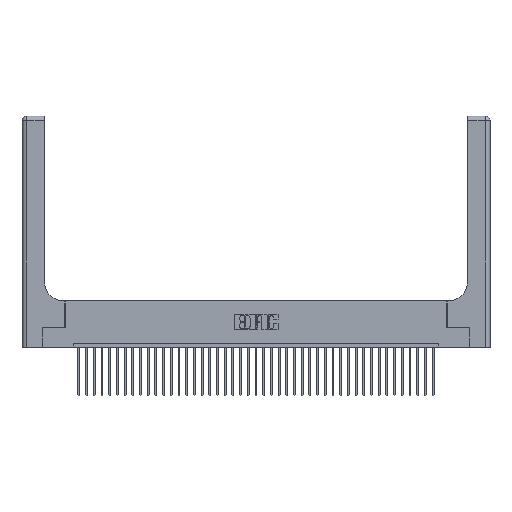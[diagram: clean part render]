
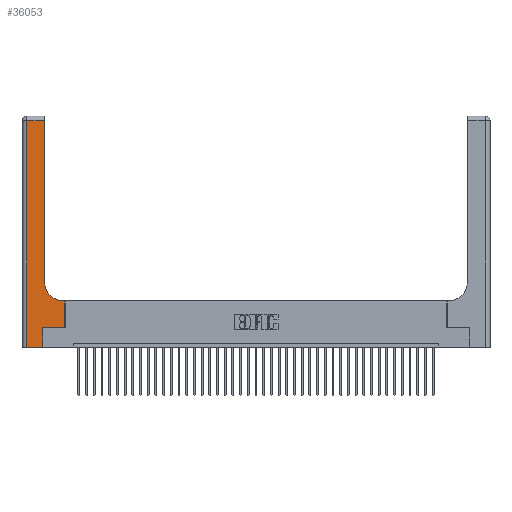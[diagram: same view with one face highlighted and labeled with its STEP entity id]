
A CAD part, top view. The second image highlights one B-rep face of the part: STEP entity #36053.
In plain terms, the highlighted planar face has unit normal (0, 0, 1).
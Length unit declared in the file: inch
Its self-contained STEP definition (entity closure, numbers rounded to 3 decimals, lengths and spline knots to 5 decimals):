
#49 = CARTESIAN_POINT ( 'NONE',  ( 0., 2.94, 0.37 ) ) ;
#161 = VERTEX_POINT ( 'NONE', #31166 ) ;
#651 = EDGE_CURVE ( 'NONE', #8113, #23962, #15244, .T. ) ;
#875 = CARTESIAN_POINT ( 'NONE',  ( 0., 0., 0.37 ) ) ;
#1107 = LINE ( 'NONE', #34322, #7401 ) ;
#2987 = DIRECTION ( 'NONE',  ( 1., 0., 0. ) ) ;
#3810 = LINE ( 'NONE', #9054, #38551 ) ;
#3890 = EDGE_CURVE ( 'NONE', #18270, #8113, #21351, .T. ) ;
#4877 = EDGE_CURVE ( 'NONE', #21331, #4894, #12464, .T. ) ;
#4894 = VERTEX_POINT ( 'NONE', #25846 ) ;
#6618 = CARTESIAN_POINT ( 'NONE',  ( 0.5415, 0.85, 0.37 ) ) ;
#6692 = DIRECTION ( 'NONE',  ( 1., 0., 0. ) ) ;
#6704 = CARTESIAN_POINT ( 'NONE',  ( 0.5585, 0.25, 0.37 ) ) ;
#7362 = VECTOR ( 'NONE', #6692, 39.37008 ) ;
#7401 = VECTOR ( 'NONE', #28544, 39.37008 ) ;
#8113 = VERTEX_POINT ( 'NONE', #14712 ) ;
#8853 = FACE_OUTER_BOUND ( 'NONE', #10346, .T. ) ;
#9054 = CARTESIAN_POINT ( 'NONE',  ( 0.269, 0.25, 0.37 ) ) ;
#9971 = VERTEX_POINT ( 'NONE', #36101 ) ;
#10346 = EDGE_LOOP ( 'NONE', ( #34549, #17338, #36298, #28625, #17336, #20316, #34508, #25698, #30585 ) ) ;
#10503 = DIRECTION ( 'NONE',  ( -1., 0., 0. ) ) ;
#11169 = CARTESIAN_POINT ( 'NONE',  ( 0.269, 0., 0.37 ) ) ;
#11776 = EDGE_CURVE ( 'NONE', #9971, #32318, #22780, .T. ) ;
#12464 = LINE ( 'NONE', #6704, #35665 ) ;
#12509 = CARTESIAN_POINT ( 'NONE',  ( 0.5585, 0.25, 0.37 ) ) ;
#13069 = DIRECTION ( 'NONE',  ( 0., 0., -1. ) ) ;
#14148 = DIRECTION ( 'NONE',  ( 0., 1., 0. ) ) ;
#14547 = CARTESIAN_POINT ( 'NONE',  ( 0.2915, 2.94, 0.37 ) ) ;
#14557 = VECTOR ( 'NONE', #10503, 39.37008 ) ;
#14712 = CARTESIAN_POINT ( 'NONE',  ( 0.06, 2.94, 0.37 ) ) ;
#15244 = LINE ( 'NONE', #39171, #17190 ) ;
#15920 = DIRECTION ( 'NONE',  ( 0., 1., 0. ) ) ;
#17190 = VECTOR ( 'NONE', #17551, 39.37008 ) ;
#17336 = ORIENTED_EDGE ( 'NONE', *, *, #11776, .T. ) ;
#17338 = ORIENTED_EDGE ( 'NONE', *, *, #3890, .T. ) ;
#17534 = CARTESIAN_POINT ( 'NONE',  ( 0.269, 0.25, 0.37 ) ) ;
#17551 = DIRECTION ( 'NONE',  ( 0., -1., 0. ) ) ;
#18270 = VERTEX_POINT ( 'NONE', #14547 ) ;
#19774 = CARTESIAN_POINT ( 'NONE',  ( 0., 3., 0.37 ) ) ;
#20312 = VECTOR ( 'NONE', #22445, 39.37008 ) ;
#20316 = ORIENTED_EDGE ( 'NONE', *, *, #36431, .T. ) ;
#20877 = EDGE_CURVE ( 'NONE', #23962, #9971, #24330, .T. ) ;
#21331 = VERTEX_POINT ( 'NONE', #12509 ) ;
#21351 = LINE ( 'NONE', #49, #14557 ) ;
#22445 = DIRECTION ( 'NONE',  ( 0., 1., 0. ) ) ;
#22780 = LINE ( 'NONE', #11169, #35804 ) ;
#22971 = AXIS2_PLACEMENT_3D ( 'NONE', #6618, #13069, #28205 ) ;
#23962 = VERTEX_POINT ( 'NONE', #29622 ) ;
#24330 = LINE ( 'NONE', #875, #7362 ) ;
#24387 = EDGE_CURVE ( 'NONE', #4894, #36514, #1107, .T. ) ;
#25698 = ORIENTED_EDGE ( 'NONE', *, *, #24387, .T. ) ;
#25846 = CARTESIAN_POINT ( 'NONE',  ( 0.5585, 0.6, 0.37 ) ) ;
#26446 = EDGE_CURVE ( 'NONE', #161, #18270, #38524, .T. ) ;
#27929 = CARTESIAN_POINT ( 'NONE',  ( 0.5415, 0.6, 0.37 ) ) ;
#28205 = DIRECTION ( 'NONE',  ( 1., 0., 0. ) ) ;
#28544 = DIRECTION ( 'NONE',  ( -1., 0., 0. ) ) ;
#28625 = ORIENTED_EDGE ( 'NONE', *, *, #20877, .T. ) ;
#28633 = PLANE ( 'NONE',  #38048 ) ;
#28774 = DIRECTION ( 'NONE',  ( 0., 0., -1. ) ) ;
#28905 = CARTESIAN_POINT ( 'NONE',  ( 0.2915, 3., 0.37 ) ) ;
#29622 = CARTESIAN_POINT ( 'NONE',  ( 0.06, 0., 0.37 ) ) ;
#29813 = CIRCLE ( 'NONE', #22971, 0.25 ) ;
#30585 = ORIENTED_EDGE ( 'NONE', *, *, #39046, .T. ) ;
#31166 = CARTESIAN_POINT ( 'NONE',  ( 0.2915, 0.85, 0.37 ) ) ;
#32318 = VERTEX_POINT ( 'NONE', #17534 ) ;
#34322 = CARTESIAN_POINT ( 'NONE',  ( 0.2915, 0.6, 0.37 ) ) ;
#34508 = ORIENTED_EDGE ( 'NONE', *, *, #4877, .T. ) ;
#34549 = ORIENTED_EDGE ( 'NONE', *, *, #26446, .T. ) ;
#34811 = DIRECTION ( 'NONE',  ( -1., 0., 0. ) ) ;
#35665 = VECTOR ( 'NONE', #15920, 39.37008 ) ;
#35804 = VECTOR ( 'NONE', #14148, 39.37008 ) ;
#36053 = ADVANCED_FACE ( 'NONE', ( #8853 ), #28633, .F. ) ;
#36101 = CARTESIAN_POINT ( 'NONE',  ( 0.269, 0., 0.37 ) ) ;
#36298 = ORIENTED_EDGE ( 'NONE', *, *, #651, .T. ) ;
#36431 = EDGE_CURVE ( 'NONE', #32318, #21331, #3810, .T. ) ;
#36514 = VERTEX_POINT ( 'NONE', #27929 ) ;
#38048 = AXIS2_PLACEMENT_3D ( 'NONE', #19774, #28774, #34811 ) ;
#38524 = LINE ( 'NONE', #28905, #20312 ) ;
#38551 = VECTOR ( 'NONE', #2987, 39.37008 ) ;
#39046 = EDGE_CURVE ( 'NONE', #36514, #161, #29813, .T. ) ;
#39171 = CARTESIAN_POINT ( 'NONE',  ( 0.06, 3., 0.37 ) ) ;
